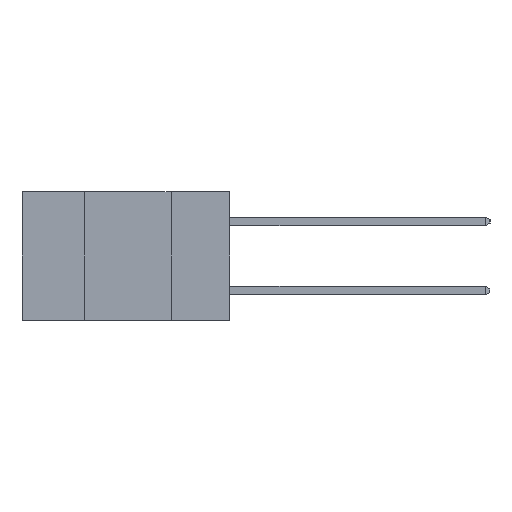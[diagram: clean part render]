
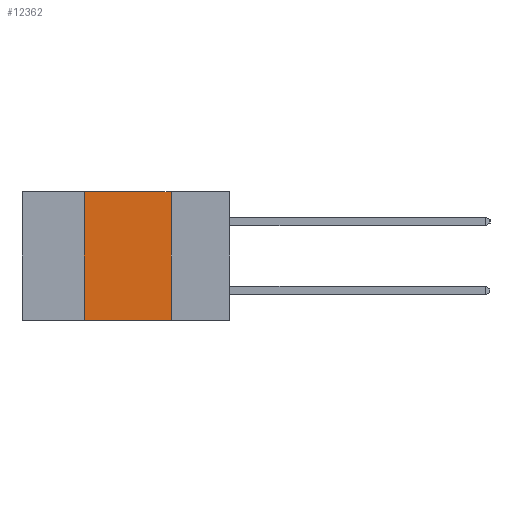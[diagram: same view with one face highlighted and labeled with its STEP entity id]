
A CAD part, left-side view. The second image highlights one B-rep face of the part: STEP entity #12362.
In plain terms, the highlighted planar face has unit normal (-1, 0, 0).
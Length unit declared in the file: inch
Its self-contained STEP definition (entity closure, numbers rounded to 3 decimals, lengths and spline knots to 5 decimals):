
#370 = EDGE_CURVE ( 'NONE', #12148, #948, #15784, .T. ) ;
#564 = FACE_OUTER_BOUND ( 'NONE', #10632, .T. ) ;
#721 = CARTESIAN_POINT ( 'NONE',  ( 0., 0.42, 0. ) ) ;
#948 = VERTEX_POINT ( 'NONE', #721 ) ;
#1817 = ORIENTED_EDGE ( 'NONE', *, *, #2010, .F. ) ;
#1831 = DIRECTION ( 'NONE',  ( 0., 0., 1. ) ) ;
#2010 = EDGE_CURVE ( 'NONE', #16340, #15754, #18456, .T. ) ;
#2583 = CARTESIAN_POINT ( 'NONE',  ( 0., 0.42, 0. ) ) ;
#2773 = ORIENTED_EDGE ( 'NONE', *, *, #7310, .F. ) ;
#4812 = CARTESIAN_POINT ( 'NONE',  ( 0., 0.17, 0. ) ) ;
#5581 = DIRECTION ( 'NONE',  ( 1., 0., 0. ) ) ;
#6653 = CARTESIAN_POINT ( 'NONE',  ( 0., 0.42, -0.37 ) ) ;
#7310 = EDGE_CURVE ( 'NONE', #948, #16340, #9456, .T. ) ;
#7419 = VECTOR ( 'NONE', #1831, 39.37008 ) ;
#8187 = AXIS2_PLACEMENT_3D ( 'NONE', #14910, #5581, #16531 ) ;
#8598 = PLANE ( 'NONE',  #8187 ) ;
#9254 = EDGE_CURVE ( 'NONE', #12148, #15754, #19723, .T. ) ;
#9456 = LINE ( 'NONE', #12593, #13137 ) ;
#10247 = CARTESIAN_POINT ( 'NONE',  ( 0., 0.6, -0.37 ) ) ;
#10632 = EDGE_LOOP ( 'NONE', ( #1817, #2773, #15685, #18166 ) ) ;
#11791 = DIRECTION ( 'NONE',  ( 0., -1., 0. ) ) ;
#12148 = VERTEX_POINT ( 'NONE', #6653 ) ;
#12362 = ADVANCED_FACE ( 'NONE', ( #564 ), #8598, .F. ) ;
#12593 = CARTESIAN_POINT ( 'NONE',  ( 0., 0.6, 0. ) ) ;
#13137 = VECTOR ( 'NONE', #14206, 39.37008 ) ;
#14206 = DIRECTION ( 'NONE',  ( 0., -1., 0. ) ) ;
#14251 = VECTOR ( 'NONE', #16679, 39.37008 ) ;
#14489 = CARTESIAN_POINT ( 'NONE',  ( 0., 0.17, -0.37 ) ) ;
#14910 = CARTESIAN_POINT ( 'NONE',  ( 0., 0.6, 0. ) ) ;
#15685 = ORIENTED_EDGE ( 'NONE', *, *, #370, .F. ) ;
#15754 = VERTEX_POINT ( 'NONE', #14489 ) ;
#15784 = LINE ( 'NONE', #2583, #7419 ) ;
#15944 = CARTESIAN_POINT ( 'NONE',  ( 0., 0.17, 0. ) ) ;
#16340 = VERTEX_POINT ( 'NONE', #4812 ) ;
#16531 = DIRECTION ( 'NONE',  ( 0., 0., -1. ) ) ;
#16578 = VECTOR ( 'NONE', #11791, 39.37008 ) ;
#16679 = DIRECTION ( 'NONE',  ( 0., 0., -1. ) ) ;
#18166 = ORIENTED_EDGE ( 'NONE', *, *, #9254, .T. ) ;
#18456 = LINE ( 'NONE', #15944, #14251 ) ;
#19723 = LINE ( 'NONE', #10247, #16578 ) ;
